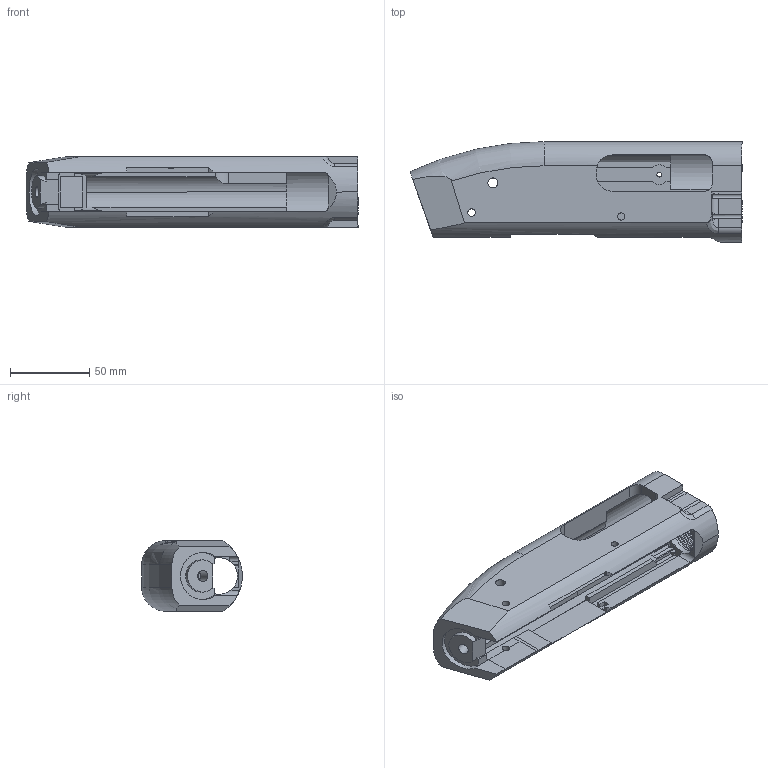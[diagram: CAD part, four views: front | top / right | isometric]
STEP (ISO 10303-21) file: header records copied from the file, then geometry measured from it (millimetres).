
FILE_DESCRIPTION(('FreeCAD Model'),'2;1');
FILE_NAME('Open CASCADE Shape Model','2024-11-03T13:24:41',(''),(''), 'Open CASCADE STEP processor 7.6','FreeCAD','Unknown');
FILE_SCHEMA(('AUTOMOTIVE_DESIGN { 1 0 10303 214 1 1 1 1 }'));
Length unit declared in the file: millimetre
Products named in the file (1): Pocket033
Bounding box: 209.55 x 63.5 x 44.45 mm (x, y, z)
Volume: 197176.1 mm3; surface area: 66292.6 mm2
Topology: 1 solids, 1 shells, 241 faces, 709 edges, 463 vertices
Faces by surface type: plane 157, cylinder 59, bspline 23, torus 2
Full cylindrical faces by diameter (mm): 3.048 x1, 3.175 x2, 4.572 x1, 4.826 x2, 6.35 x2, 6.858 x1, 23.114 x1, 24.384 x6, 32.766 x1
Entity records: 26783 total; most frequent: CARTESIAN_POINT 13840, DIRECTION 2040, ORIENTED_EDGE 1418, PCURVE 1418, DEFINITIONAL_REPRESENTATION 1418, LINE 1226, VECTOR 1226, EDGE_CURVE 709
